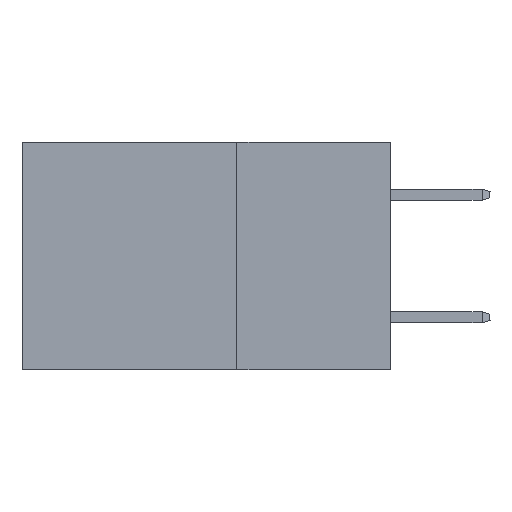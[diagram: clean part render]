
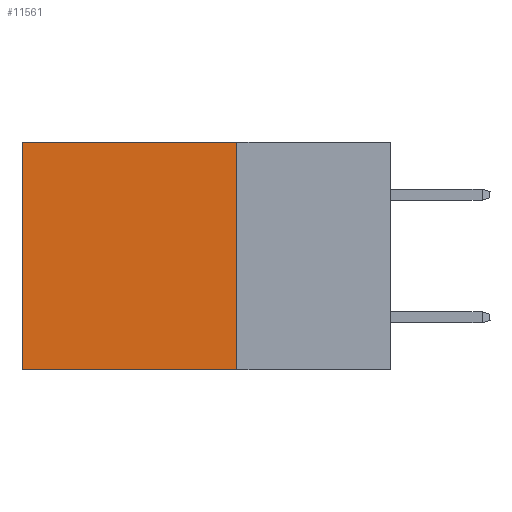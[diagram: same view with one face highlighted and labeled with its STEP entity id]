
A CAD part, left-side view. The second image highlights one B-rep face of the part: STEP entity #11561.
In plain terms, the highlighted planar face has unit normal (-1, 0, 0).
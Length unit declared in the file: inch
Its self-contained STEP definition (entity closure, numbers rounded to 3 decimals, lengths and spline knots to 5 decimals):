
#98 = DIRECTION ( 'NONE',  ( 0., 0., -1. ) ) ;
#837 = EDGE_CURVE ( 'NONE', #34021, #27405, #15810, .T. ) ;
#1378 = EDGE_LOOP ( 'NONE', ( #11126, #22573, #18435, #20070 ) ) ;
#4990 = CARTESIAN_POINT ( 'NONE',  ( 0.2875, 0.6, 0. ) ) ;
#7797 = VECTOR ( 'NONE', #27104, 39.37008 ) ;
#8771 = CARTESIAN_POINT ( 'NONE',  ( 0.2875, 0.25, -0.37 ) ) ;
#9412 = CARTESIAN_POINT ( 'NONE',  ( 0.2875, 0.6, -0.37 ) ) ;
#11126 = ORIENTED_EDGE ( 'NONE', *, *, #16932, .T. ) ;
#11561 = ADVANCED_FACE ( 'NONE', ( #21761 ), #14286, .F. ) ;
#13906 = DIRECTION ( 'NONE',  ( 0., 0., -1. ) ) ;
#14286 = PLANE ( 'NONE',  #17419 ) ;
#15810 = LINE ( 'NONE', #23354, #7797 ) ;
#16932 = EDGE_CURVE ( 'NONE', #27405, #19541, #25847, .T. ) ;
#17053 = DIRECTION ( 'NONE',  ( 1., 0., 0. ) ) ;
#17419 = AXIS2_PLACEMENT_3D ( 'NONE', #29144, #17053, #13906 ) ;
#18435 = ORIENTED_EDGE ( 'NONE', *, *, #34803, .F. ) ;
#19422 = EDGE_CURVE ( 'NONE', #34447, #19541, #28788, .T. ) ;
#19541 = VERTEX_POINT ( 'NONE', #9412 ) ;
#20070 = ORIENTED_EDGE ( 'NONE', *, *, #837, .T. ) ;
#21761 = FACE_OUTER_BOUND ( 'NONE', #1378, .T. ) ;
#22573 = ORIENTED_EDGE ( 'NONE', *, *, #19422, .F. ) ;
#23354 = CARTESIAN_POINT ( 'NONE',  ( 0.2875, 0.25, 0. ) ) ;
#25108 = DIRECTION ( 'NONE',  ( 0., 0., -1. ) ) ;
#25847 = LINE ( 'NONE', #36073, #35163 ) ;
#27104 = DIRECTION ( 'NONE',  ( 0., 1., 0. ) ) ;
#27405 = VERTEX_POINT ( 'NONE', #4990 ) ;
#27833 = CARTESIAN_POINT ( 'NONE',  ( 0.2875, 0.25, 0. ) ) ;
#28788 = LINE ( 'NONE', #32728, #38621 ) ;
#29144 = CARTESIAN_POINT ( 'NONE',  ( 0.2875, 0.25, 0. ) ) ;
#32618 = VECTOR ( 'NONE', #25108, 39.37008 ) ;
#32728 = CARTESIAN_POINT ( 'NONE',  ( 0.2875, 0.25, -0.37 ) ) ;
#34021 = VERTEX_POINT ( 'NONE', #36622 ) ;
#34447 = VERTEX_POINT ( 'NONE', #8771 ) ;
#34803 = EDGE_CURVE ( 'NONE', #34021, #34447, #35860, .T. ) ;
#35163 = VECTOR ( 'NONE', #98, 39.37008 ) ;
#35860 = LINE ( 'NONE', #27833, #32618 ) ;
#36073 = CARTESIAN_POINT ( 'NONE',  ( 0.2875, 0.6, 0. ) ) ;
#36622 = CARTESIAN_POINT ( 'NONE',  ( 0.2875, 0.25, 0. ) ) ;
#38222 = DIRECTION ( 'NONE',  ( 0., 1., 0. ) ) ;
#38621 = VECTOR ( 'NONE', #38222, 39.37008 ) ;
